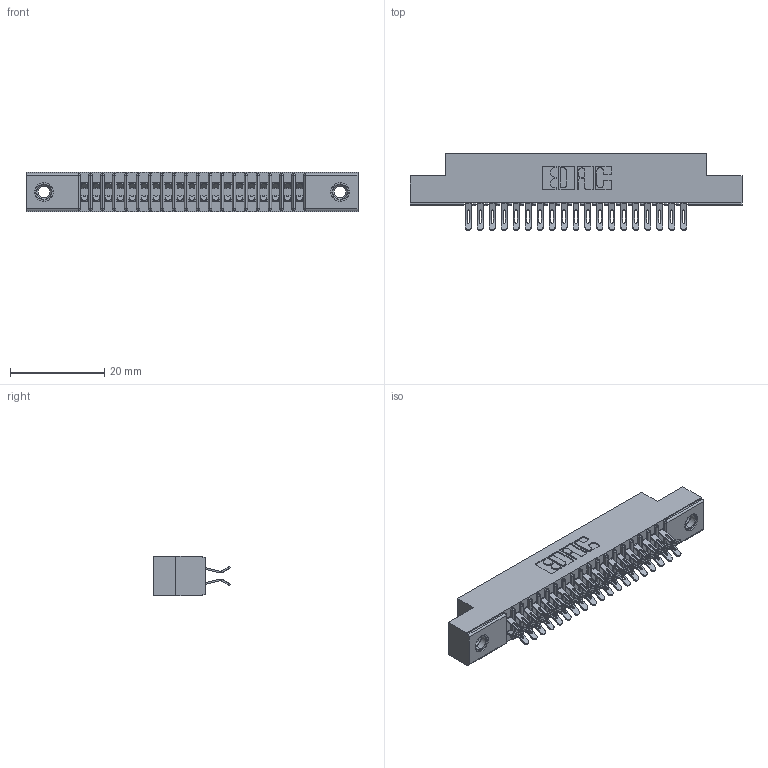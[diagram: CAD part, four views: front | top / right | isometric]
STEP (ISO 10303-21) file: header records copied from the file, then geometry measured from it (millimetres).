
FILE_DESCRIPTION (( 'STEP AP203' ), '1' );
FILE_NAME ('391-038-555-207.STEP', '2018-08-09T00:21:10', ( '' ), ( '' ), 'SwSTEP 2.0', 'SolidWorks 2016', '' );
FILE_SCHEMA (( 'CONFIG_CONTROL_DESIGN' ));
Length unit declared in the file: inch
Products named in the file (4): 391-038-555-207; 341 Part_.156 (3.96) Dia Mounting Holes; 341-292-001_341-292-155; 345-250-001_345-250-005-103
Assembly tree (41 placements, depth 2):
  391-038-555-207
    341 Part_.156 (3.96) Dia Mounting Holes
    341-292-001_341-292-155  x38
    345-250-001_345-250-005-103  x2
Bounding box: 70.48 x 16.31 x 8.38 mm (x, y, z)
Volume: 4055.8 mm3; surface area: 8597.1 mm2
Topology: 41 solids, 41 shells, 3140 faces, 9325 edges, 6066 vertices
Faces by surface type: plane 1696, cylinder 1352, sphere 40, torus 40, cone 12
Entity records: 27713 total; most frequent: CARTESIAN_POINT 4606, ORIENTED_EDGE 4558, DIRECTION 4487, EDGE_CURVE 2279, LINE 1797, VECTOR 1797, VERTEX_POINT 1448, AXIS2_PLACEMENT_3D 1345
